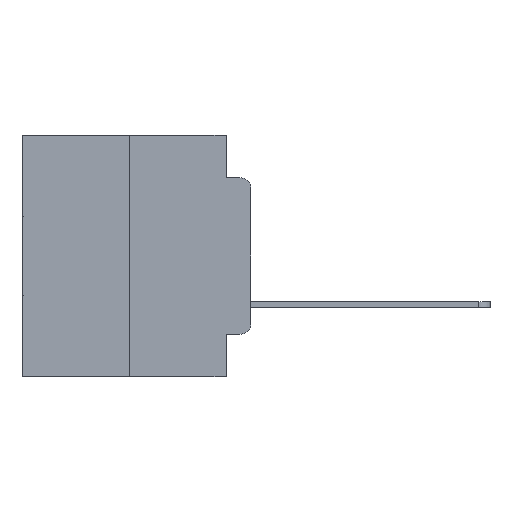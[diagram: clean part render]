
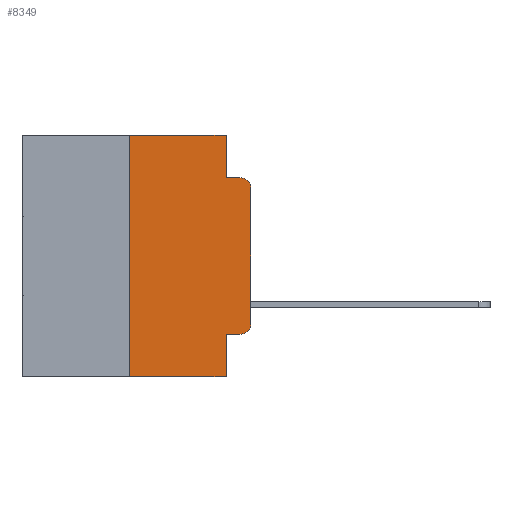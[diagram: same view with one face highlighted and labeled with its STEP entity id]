
A CAD part, left-side view. The second image highlights one B-rep face of the part: STEP entity #8349.
In plain terms, the highlighted planar face has unit normal (-1, 0, 0).
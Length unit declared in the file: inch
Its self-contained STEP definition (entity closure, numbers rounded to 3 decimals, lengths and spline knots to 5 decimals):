
#596 = ORIENTED_EDGE ( 'NONE', *, *, #30816, .T. ) ;
#854 = DIRECTION ( 'NONE',  ( 0., 0., 1. ) ) ;
#1056 = EDGE_CURVE ( 'NONE', #29471, #3557, #5328, .T. ) ;
#1291 = CARTESIAN_POINT ( 'NONE',  ( 0., 0.02, -0.4115 ) ) ;
#1648 = ORIENTED_EDGE ( 'NONE', *, *, #10183, .F. ) ;
#2234 = EDGE_CURVE ( 'NONE', #13504, #17153, #10952, .T. ) ;
#2358 = ORIENTED_EDGE ( 'NONE', *, *, #2921, .T. ) ;
#2811 = ORIENTED_EDGE ( 'NONE', *, *, #1056, .T. ) ;
#2877 = VERTEX_POINT ( 'NONE', #30335 ) ;
#2921 = EDGE_CURVE ( 'NONE', #25464, #29471, #10846, .T. ) ;
#3032 = LINE ( 'NONE', #8265, #15896 ) ;
#3552 = ORIENTED_EDGE ( 'NONE', *, *, #13913, .F. ) ;
#3557 = VERTEX_POINT ( 'NONE', #24991 ) ;
#5328 = CIRCLE ( 'NONE', #23689, 0.02 ) ;
#6006 = EDGE_CURVE ( 'NONE', #3557, #13504, #6405, .T. ) ;
#6405 = LINE ( 'NONE', #7400, #29799 ) ;
#7400 = CARTESIAN_POINT ( 'NONE',  ( 0., 0., 0. ) ) ;
#7730 = LINE ( 'NONE', #29738, #9435 ) ;
#7797 = AXIS2_PLACEMENT_3D ( 'NONE', #28473, #26212, #19560 ) ;
#8124 = VECTOR ( 'NONE', #15594, 39.37008 ) ;
#8265 = CARTESIAN_POINT ( 'NONE',  ( 0., 0.051, 0. ) ) ;
#8349 = ADVANCED_FACE ( 'NONE', ( #20713 ), #17274, .F. ) ;
#9404 = DIRECTION ( 'NONE',  ( -1., 0., 0. ) ) ;
#9435 = VECTOR ( 'NONE', #854, 39.37008 ) ;
#10183 = EDGE_CURVE ( 'NONE', #25464, #17016, #19860, .T. ) ;
#10643 = ORIENTED_EDGE ( 'NONE', *, *, #6006, .T. ) ;
#10846 = LINE ( 'NONE', #28327, #22500 ) ;
#10893 = DIRECTION ( 'NONE',  ( 0., 0., -1. ) ) ;
#10952 = CIRCLE ( 'NONE', #14573, 0.02 ) ;
#11891 = EDGE_CURVE ( 'NONE', #25177, #22433, #7730, .T. ) ;
#12883 = CARTESIAN_POINT ( 'NONE',  ( 0., 0.25, 0. ) ) ;
#12929 = ORIENTED_EDGE ( 'NONE', *, *, #2234, .T. ) ;
#13186 = VERTEX_POINT ( 'NONE', #18478 ) ;
#13504 = VERTEX_POINT ( 'NONE', #16954 ) ;
#13775 = VECTOR ( 'NONE', #15939, 39.37008 ) ;
#13913 = EDGE_CURVE ( 'NONE', #22433, #2877, #26705, .T. ) ;
#14036 = ORIENTED_EDGE ( 'NONE', *, *, #30092, .F. ) ;
#14169 = CARTESIAN_POINT ( 'NONE',  ( 0., 0.25, -0.5 ) ) ;
#14573 = AXIS2_PLACEMENT_3D ( 'NONE', #23444, #9404, #25683 ) ;
#15392 = ORIENTED_EDGE ( 'NONE', *, *, #24260, .F. ) ;
#15594 = DIRECTION ( 'NONE',  ( 0., -1., 0. ) ) ;
#15879 = DIRECTION ( 'NONE',  ( 0., 0., -1. ) ) ;
#15896 = VECTOR ( 'NONE', #10893, 39.37008 ) ;
#15939 = DIRECTION ( 'NONE',  ( 0., 0., -1. ) ) ;
#16954 = CARTESIAN_POINT ( 'NONE',  ( 0., 0., -0.1085 ) ) ;
#17016 = VERTEX_POINT ( 'NONE', #23360 ) ;
#17153 = VERTEX_POINT ( 'NONE', #28125 ) ;
#17274 = PLANE ( 'NONE',  #7797 ) ;
#17318 = DIRECTION ( 'NONE',  ( 0., 0., 1. ) ) ;
#17876 = CARTESIAN_POINT ( 'NONE',  ( 0., 0.051, -0.4115 ) ) ;
#17949 = DIRECTION ( 'NONE',  ( 0., -1., 0. ) ) ;
#18478 = CARTESIAN_POINT ( 'NONE',  ( 0., 0.051, -0.0885 ) ) ;
#19560 = DIRECTION ( 'NONE',  ( 0., 0., -1. ) ) ;
#19860 = LINE ( 'NONE', #22711, #13775 ) ;
#20713 = FACE_OUTER_BOUND ( 'NONE', #24550, .T. ) ;
#20787 = VECTOR ( 'NONE', #17949, 39.37008 ) ;
#20833 = CARTESIAN_POINT ( 'NONE',  ( 0., 0.02, -0.3915 ) ) ;
#20897 = DIRECTION ( 'NONE',  ( -1., 0., 0. ) ) ;
#20977 = ORIENTED_EDGE ( 'NONE', *, *, #11891, .F. ) ;
#22433 = VERTEX_POINT ( 'NONE', #12883 ) ;
#22500 = VECTOR ( 'NONE', #26068, 39.37008 ) ;
#22711 = CARTESIAN_POINT ( 'NONE',  ( 0., 0.051, 0. ) ) ;
#23360 = CARTESIAN_POINT ( 'NONE',  ( 0., 0.051, -0.5 ) ) ;
#23444 = CARTESIAN_POINT ( 'NONE',  ( 0., 0.02, -0.1085 ) ) ;
#23689 = AXIS2_PLACEMENT_3D ( 'NONE', #20833, #20897, #15879 ) ;
#24260 = EDGE_CURVE ( 'NONE', #2877, #13186, #3032, .T. ) ;
#24527 = CARTESIAN_POINT ( 'NONE',  ( 0., 0.473, -0.5 ) ) ;
#24550 = EDGE_LOOP ( 'NONE', ( #10643, #12929, #14036, #15392, #3552, #20977, #596, #1648, #2358, #2811 ) ) ;
#24991 = CARTESIAN_POINT ( 'NONE',  ( 0., 0., -0.3915 ) ) ;
#25177 = VERTEX_POINT ( 'NONE', #14169 ) ;
#25464 = VERTEX_POINT ( 'NONE', #17876 ) ;
#25683 = DIRECTION ( 'NONE',  ( 0., 0., -1. ) ) ;
#26068 = DIRECTION ( 'NONE',  ( 0., -1., 0. ) ) ;
#26212 = DIRECTION ( 'NONE',  ( 1., 0., 0. ) ) ;
#26425 = VECTOR ( 'NONE', #26727, 39.37008 ) ;
#26705 = LINE ( 'NONE', #26870, #20787 ) ;
#26727 = DIRECTION ( 'NONE',  ( 0., -1., 0. ) ) ;
#26807 = LINE ( 'NONE', #26858, #8124 ) ;
#26858 = CARTESIAN_POINT ( 'NONE',  ( 0., 0.051, -0.0885 ) ) ;
#26870 = CARTESIAN_POINT ( 'NONE',  ( 0., 0.473, 0. ) ) ;
#27131 = LINE ( 'NONE', #24527, #26425 ) ;
#28125 = CARTESIAN_POINT ( 'NONE',  ( 0., 0.02, -0.0885 ) ) ;
#28327 = CARTESIAN_POINT ( 'NONE',  ( 0., 0.051, -0.4115 ) ) ;
#28473 = CARTESIAN_POINT ( 'NONE',  ( 0., 0.473, 0. ) ) ;
#29471 = VERTEX_POINT ( 'NONE', #1291 ) ;
#29738 = CARTESIAN_POINT ( 'NONE',  ( 0., 0.25, 0. ) ) ;
#29799 = VECTOR ( 'NONE', #17318, 39.37008 ) ;
#30092 = EDGE_CURVE ( 'NONE', #13186, #17153, #26807, .T. ) ;
#30335 = CARTESIAN_POINT ( 'NONE',  ( 0., 0.051, 0. ) ) ;
#30816 = EDGE_CURVE ( 'NONE', #25177, #17016, #27131, .T. ) ;
